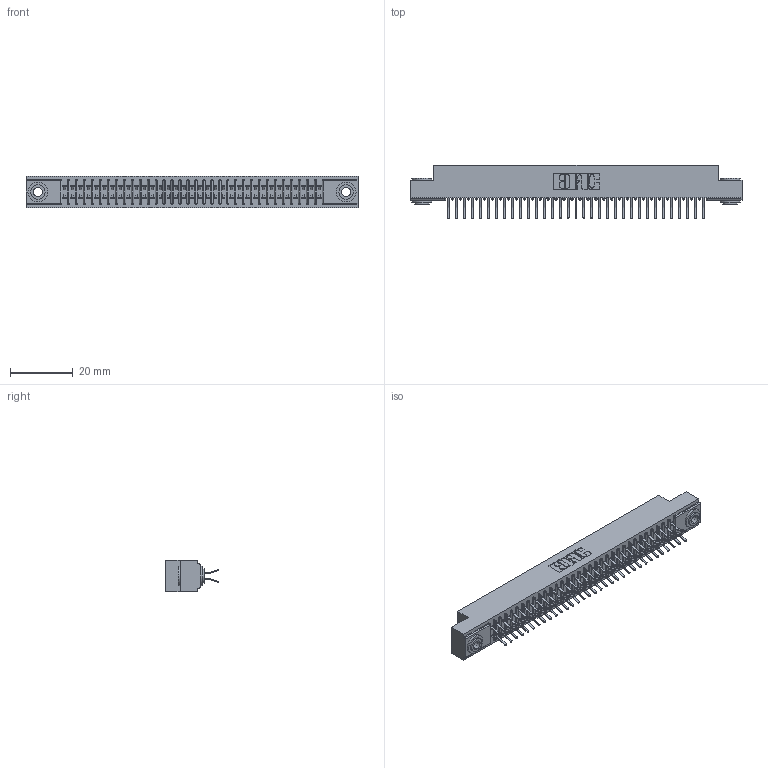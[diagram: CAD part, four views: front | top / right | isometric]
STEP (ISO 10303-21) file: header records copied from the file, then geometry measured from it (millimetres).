
FILE_DESCRIPTION (( 'STEP AP203' ), '1' );
FILE_NAME ('391-066-556-203.STEP', '2018-08-09T13:35:42', ( '' ), ( '' ), 'SwSTEP 2.0', 'SolidWorks 2016', '' );
FILE_SCHEMA (( 'CONFIG_CONTROL_DESIGN' ));
Length unit declared in the file: inch
Products named in the file (4): 341-292-001_341-292-156; 345-250-002_345-250-002-102; 391-066-556-203; 341 Part_.156 (3.96) Dia Mounting Holes
Assembly tree (69 placements, depth 2):
  391-066-556-203
    341 Part_.156 (3.96) Dia Mounting Holes
    341-292-001_341-292-156  x66
    345-250-002_345-250-002-102  x2
Bounding box: 106.05 x 17.07 x 10.16 mm (x, y, z)
Volume: 7845.3 mm3; surface area: 14044.3 mm2
Topology: 69 solids, 69 shells, 4788 faces, 13859 edges, 8990 vertices
Faces by surface type: plane 2732, cylinder 1916, sphere 68, torus 64, cone 8
Entity records: 42341 total; most frequent: CARTESIAN_POINT 7020, ORIENTED_EDGE 6966, DIRECTION 6839, EDGE_CURVE 3483, VECTOR 2789, LINE 2789, VERTEX_POINT 2206, AXIS2_PLACEMENT_3D 2025
